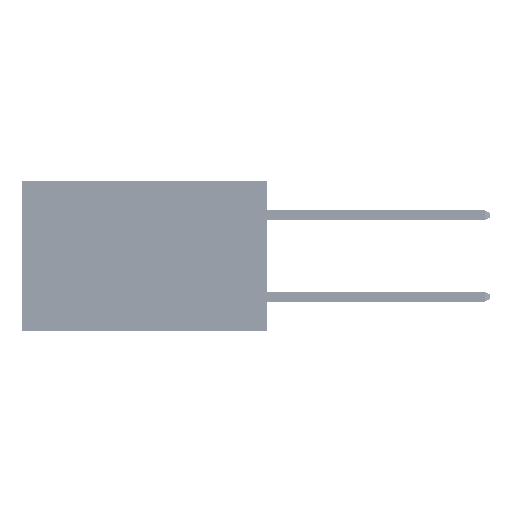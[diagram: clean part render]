
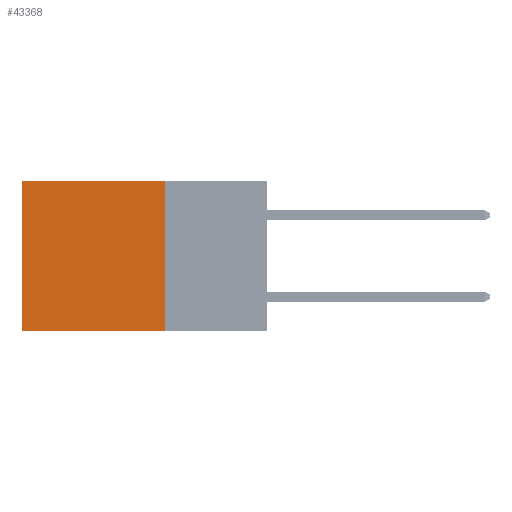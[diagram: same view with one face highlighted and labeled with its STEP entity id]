
A CAD part, left-side view. The second image highlights one B-rep face of the part: STEP entity #43368.
In plain terms, the highlighted planar face has unit normal (-1, 0, 0).
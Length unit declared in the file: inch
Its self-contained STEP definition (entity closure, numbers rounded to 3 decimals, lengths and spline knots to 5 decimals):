
#144 = CARTESIAN_POINT ( 'NONE',  ( 0.2875, 0.25, 0. ) ) ;
#3315 = VERTEX_POINT ( 'NONE', #46192 ) ;
#3516 = LINE ( 'NONE', #34049, #44376 ) ;
#5447 = CARTESIAN_POINT ( 'NONE',  ( 0.2875, 0.25, 0. ) ) ;
#7771 = AXIS2_PLACEMENT_3D ( 'NONE', #144, #50214, #18997 ) ;
#8700 = VERTEX_POINT ( 'NONE', #17864 ) ;
#12267 = ORIENTED_EDGE ( 'NONE', *, *, #39021, .F. ) ;
#13461 = DIRECTION ( 'NONE',  ( 0., 0., -1. ) ) ;
#17864 = CARTESIAN_POINT ( 'NONE',  ( 0.2875, 0.25, -0.37 ) ) ;
#18997 = DIRECTION ( 'NONE',  ( 0., 0., -1. ) ) ;
#19957 = FACE_OUTER_BOUND ( 'NONE', #29105, .T. ) ;
#20713 = EDGE_CURVE ( 'NONE', #31618, #30380, #45252, .T. ) ;
#21762 = LINE ( 'NONE', #48901, #24187 ) ;
#23146 = EDGE_CURVE ( 'NONE', #8700, #3315, #3516, .T. ) ;
#24187 = VECTOR ( 'NONE', #13461, 39.37008 ) ;
#24964 = DIRECTION ( 'NONE',  ( 0., 0., -1. ) ) ;
#29105 = EDGE_LOOP ( 'NONE', ( #48274, #42091, #12267, #44653 ) ) ;
#30380 = VERTEX_POINT ( 'NONE', #44605 ) ;
#31618 = VERTEX_POINT ( 'NONE', #48488 ) ;
#31633 = CARTESIAN_POINT ( 'NONE',  ( 0.2875, 0.25, 0. ) ) ;
#34049 = CARTESIAN_POINT ( 'NONE',  ( 0.2875, 0.25, -0.37 ) ) ;
#34815 = VECTOR ( 'NONE', #36242, 39.37008 ) ;
#35073 = VECTOR ( 'NONE', #24964, 39.37008 ) ;
#36242 = DIRECTION ( 'NONE',  ( 0., 1., 0. ) ) ;
#39021 = EDGE_CURVE ( 'NONE', #31618, #8700, #45509, .T. ) ;
#42091 = ORIENTED_EDGE ( 'NONE', *, *, #23146, .F. ) ;
#42390 = PLANE ( 'NONE',  #7771 ) ;
#43368 = ADVANCED_FACE ( 'NONE', ( #19957 ), #42390, .F. ) ;
#44376 = VECTOR ( 'NONE', #49275, 39.37008 ) ;
#44605 = CARTESIAN_POINT ( 'NONE',  ( 0.2875, 0.6, 0. ) ) ;
#44653 = ORIENTED_EDGE ( 'NONE', *, *, #20713, .T. ) ;
#45252 = LINE ( 'NONE', #31633, #34815 ) ;
#45509 = LINE ( 'NONE', #5447, #35073 ) ;
#46192 = CARTESIAN_POINT ( 'NONE',  ( 0.2875, 0.6, -0.37 ) ) ;
#48274 = ORIENTED_EDGE ( 'NONE', *, *, #50366, .T. ) ;
#48488 = CARTESIAN_POINT ( 'NONE',  ( 0.2875, 0.25, 0. ) ) ;
#48901 = CARTESIAN_POINT ( 'NONE',  ( 0.2875, 0.6, 0. ) ) ;
#49275 = DIRECTION ( 'NONE',  ( 0., 1., 0. ) ) ;
#50214 = DIRECTION ( 'NONE',  ( 1., 0., 0. ) ) ;
#50366 = EDGE_CURVE ( 'NONE', #30380, #3315, #21762, .T. ) ;
